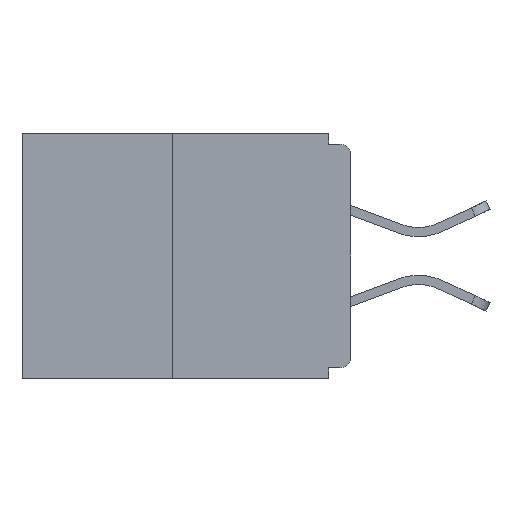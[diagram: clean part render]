
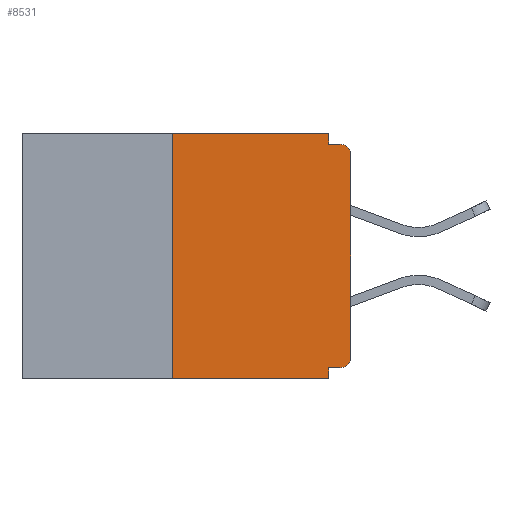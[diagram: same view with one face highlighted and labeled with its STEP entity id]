
A CAD part, left-side view. The second image highlights one B-rep face of the part: STEP entity #8531.
In plain terms, the highlighted planar face has unit normal (-1, 0, 0).
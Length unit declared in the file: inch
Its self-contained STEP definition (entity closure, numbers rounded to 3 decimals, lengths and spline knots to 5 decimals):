
#86 = LINE ( 'NONE', #3817, #10313 ) ;
#566 = ORIENTED_EDGE ( 'NONE', *, *, #8711, .F. ) ;
#567 = EDGE_CURVE ( 'NONE', #5494, #9069, #9820, .T. ) ;
#916 = VERTEX_POINT ( 'NONE', #10184 ) ;
#1031 = DIRECTION ( 'NONE',  ( 0., 0., -1. ) ) ;
#1045 = EDGE_CURVE ( 'NONE', #9092, #7594, #9949, .T. ) ;
#1233 = CIRCLE ( 'NONE', #2661, 0.015 ) ;
#1291 = CARTESIAN_POINT ( 'NONE',  ( 0., 0., -0.015 ) ) ;
#1790 = VECTOR ( 'NONE', #7495, 39.37008 ) ;
#2153 = DIRECTION ( 'NONE',  ( 0., 0., 1. ) ) ;
#2193 = CARTESIAN_POINT ( 'NONE',  ( 0., 0., -0.03 ) ) ;
#2316 = ORIENTED_EDGE ( 'NONE', *, *, #9833, .T. ) ;
#2516 = VERTEX_POINT ( 'NONE', #6953 ) ;
#2566 = ORIENTED_EDGE ( 'NONE', *, *, #3762, .F. ) ;
#2661 = AXIS2_PLACEMENT_3D ( 'NONE', #11248, #3858, #1031 ) ;
#2967 = DIRECTION ( 'NONE',  ( 0., 0., -1. ) ) ;
#3662 = EDGE_CURVE ( 'NONE', #10828, #10215, #7848, .T. ) ;
#3713 = DIRECTION ( 'NONE',  ( 0., 1., 0. ) ) ;
#3749 = ORIENTED_EDGE ( 'NONE', *, *, #3662, .T. ) ;
#3757 = CARTESIAN_POINT ( 'NONE',  ( 0., 0., -0.328 ) ) ;
#3762 = EDGE_CURVE ( 'NONE', #5494, #10955, #86, .T. ) ;
#3778 = EDGE_CURVE ( 'NONE', #7955, #10828, #9306, .T. ) ;
#3783 = CARTESIAN_POINT ( 'NONE',  ( 0., 0.015, -0.03 ) ) ;
#3817 = CARTESIAN_POINT ( 'NONE',  ( 0., 0.25, 0. ) ) ;
#3858 = DIRECTION ( 'NONE',  ( -1., 0., 0. ) ) ;
#4061 = DIRECTION ( 'NONE',  ( 0., 0., 1. ) ) ;
#4205 = ORIENTED_EDGE ( 'NONE', *, *, #1045, .F. ) ;
#4537 = ORIENTED_EDGE ( 'NONE', *, *, #5235, .F. ) ;
#4627 = CARTESIAN_POINT ( 'NONE',  ( 0., 0.46, -0.343 ) ) ;
#4869 = CARTESIAN_POINT ( 'NONE',  ( 0., 0.25, -0.343 ) ) ;
#5235 = EDGE_CURVE ( 'NONE', #916, #2516, #7963, .T. ) ;
#5323 = ORIENTED_EDGE ( 'NONE', *, *, #567, .T. ) ;
#5351 = VECTOR ( 'NONE', #10542, 39.37008 ) ;
#5436 = CARTESIAN_POINT ( 'NONE',  ( 0., 0.031, 0. ) ) ;
#5494 = VERTEX_POINT ( 'NONE', #4869 ) ;
#5532 = CARTESIAN_POINT ( 'NONE',  ( 0., 0.46, 0. ) ) ;
#5765 = VECTOR ( 'NONE', #3713, 39.37008 ) ;
#5776 = CARTESIAN_POINT ( 'NONE',  ( 0., 0.031, -0.343 ) ) ;
#6614 = DIRECTION ( 'NONE',  ( -1., 0., 0. ) ) ;
#6953 = CARTESIAN_POINT ( 'NONE',  ( 0., 0.031, -0.328 ) ) ;
#7084 = AXIS2_PLACEMENT_3D ( 'NONE', #5532, #10097, #11919 ) ;
#7178 = VECTOR ( 'NONE', #9408, 39.37008 ) ;
#7495 = DIRECTION ( 'NONE',  ( 0., -1., 0. ) ) ;
#7581 = EDGE_LOOP ( 'NONE', ( #8829, #2566, #5323, #566, #4537, #2316, #10649, #3749, #11361, #4205 ) ) ;
#7594 = VERTEX_POINT ( 'NONE', #11648 ) ;
#7821 = CARTESIAN_POINT ( 'NONE',  ( 0., 0.46, 0. ) ) ;
#7848 = CIRCLE ( 'NONE', #11638, 0.015 ) ;
#7955 = VERTEX_POINT ( 'NONE', #10084 ) ;
#7963 = LINE ( 'NONE', #3757, #5765 ) ;
#8051 = VECTOR ( 'NONE', #11665, 39.37008 ) ;
#8312 = CARTESIAN_POINT ( 'NONE',  ( 0., 0.25, 0. ) ) ;
#8318 = PLANE ( 'NONE',  #7084 ) ;
#8483 = CARTESIAN_POINT ( 'NONE',  ( 0., 0.031, 0. ) ) ;
#8531 = ADVANCED_FACE ( 'NONE', ( #11888 ), #8318, .F. ) ;
#8663 = CARTESIAN_POINT ( 'NONE',  ( 0., 0., 0. ) ) ;
#8673 = DIRECTION ( 'NONE',  ( 0., 0., -1. ) ) ;
#8711 = EDGE_CURVE ( 'NONE', #2516, #9069, #9299, .T. ) ;
#8732 = EDGE_CURVE ( 'NONE', #10955, #9092, #11748, .T. ) ;
#8829 = ORIENTED_EDGE ( 'NONE', *, *, #8732, .F. ) ;
#9069 = VERTEX_POINT ( 'NONE', #11174 ) ;
#9092 = VERTEX_POINT ( 'NONE', #5436 ) ;
#9299 = LINE ( 'NONE', #5776, #11176 ) ;
#9306 = LINE ( 'NONE', #8663, #10170 ) ;
#9408 = DIRECTION ( 'NONE',  ( 0., 0., -1. ) ) ;
#9820 = LINE ( 'NONE', #4627, #1790 ) ;
#9833 = EDGE_CURVE ( 'NONE', #916, #7955, #1233, .T. ) ;
#9949 = LINE ( 'NONE', #8483, #7178 ) ;
#9972 = CARTESIAN_POINT ( 'NONE',  ( 0., 0.015, -0.015 ) ) ;
#10084 = CARTESIAN_POINT ( 'NONE',  ( 0., 0., -0.313 ) ) ;
#10097 = DIRECTION ( 'NONE',  ( 1., 0., 0. ) ) ;
#10170 = VECTOR ( 'NONE', #4061, 39.37008 ) ;
#10184 = CARTESIAN_POINT ( 'NONE',  ( 0., 0.015, -0.328 ) ) ;
#10215 = VERTEX_POINT ( 'NONE', #9972 ) ;
#10313 = VECTOR ( 'NONE', #2153, 39.37008 ) ;
#10514 = LINE ( 'NONE', #1291, #8051 ) ;
#10542 = DIRECTION ( 'NONE',  ( 0., -1., 0. ) ) ;
#10649 = ORIENTED_EDGE ( 'NONE', *, *, #3778, .T. ) ;
#10828 = VERTEX_POINT ( 'NONE', #2193 ) ;
#10955 = VERTEX_POINT ( 'NONE', #8312 ) ;
#11174 = CARTESIAN_POINT ( 'NONE',  ( 0., 0.031, -0.343 ) ) ;
#11176 = VECTOR ( 'NONE', #8673, 39.37008 ) ;
#11248 = CARTESIAN_POINT ( 'NONE',  ( 0., 0.015, -0.313 ) ) ;
#11361 = ORIENTED_EDGE ( 'NONE', *, *, #11840, .F. ) ;
#11638 = AXIS2_PLACEMENT_3D ( 'NONE', #3783, #6614, #2967 ) ;
#11648 = CARTESIAN_POINT ( 'NONE',  ( 0., 0.031, -0.015 ) ) ;
#11665 = DIRECTION ( 'NONE',  ( 0., -1., 0. ) ) ;
#11748 = LINE ( 'NONE', #7821, #5351 ) ;
#11840 = EDGE_CURVE ( 'NONE', #7594, #10215, #10514, .T. ) ;
#11888 = FACE_OUTER_BOUND ( 'NONE', #7581, .T. ) ;
#11919 = DIRECTION ( 'NONE',  ( 0., 0., -1. ) ) ;
